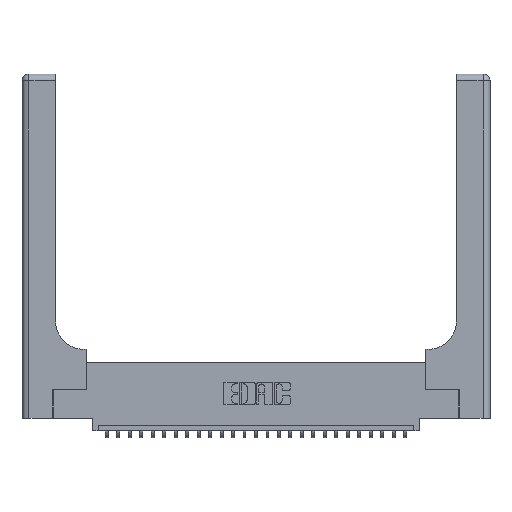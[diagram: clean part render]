
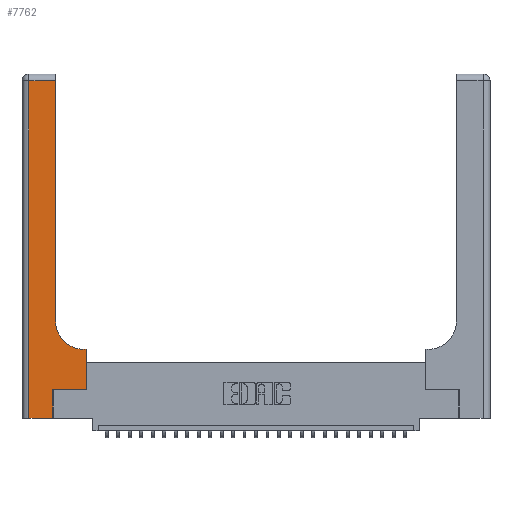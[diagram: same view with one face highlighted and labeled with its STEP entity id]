
A CAD part, top view. The second image highlights one B-rep face of the part: STEP entity #7762.
In plain terms, the highlighted planar face has unit normal (0, 0, 1).
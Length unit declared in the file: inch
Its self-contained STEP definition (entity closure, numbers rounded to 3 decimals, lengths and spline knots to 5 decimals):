
#159 = ORIENTED_EDGE ( 'NONE', *, *, #10812, .T. ) ;
#178 = LINE ( 'NONE', #2615, #13215 ) ;
#665 = ORIENTED_EDGE ( 'NONE', *, *, #11935, .T. ) ;
#1028 = VERTEX_POINT ( 'NONE', #15979 ) ;
#1153 = CARTESIAN_POINT ( 'NONE',  ( 0.2915, 0.85, 0.37 ) ) ;
#2338 = CARTESIAN_POINT ( 'NONE',  ( 0.5585, 0.25, 0.37 ) ) ;
#2615 = CARTESIAN_POINT ( 'NONE',  ( 0.269, 0.25, 0.37 ) ) ;
#2981 = AXIS2_PLACEMENT_3D ( 'NONE', #23404, #27767, #27617 ) ;
#4346 = VECTOR ( 'NONE', #11252, 39.37008 ) ;
#5257 = VERTEX_POINT ( 'NONE', #7479 ) ;
#6535 = EDGE_CURVE ( 'NONE', #14179, #15835, #25869, .T. ) ;
#7274 = ORIENTED_EDGE ( 'NONE', *, *, #15070, .T. ) ;
#7456 = CIRCLE ( 'NONE', #17212, 0.25 ) ;
#7479 = CARTESIAN_POINT ( 'NONE',  ( 0.269, 0.25, 0.37 ) ) ;
#7762 = ADVANCED_FACE ( 'NONE', ( #18041 ), #10646, .F. ) ;
#8376 = VECTOR ( 'NONE', #12177, 39.37008 ) ;
#8519 = CARTESIAN_POINT ( 'NONE',  ( 0.06, 2.94, 0.37 ) ) ;
#8842 = DIRECTION ( 'NONE',  ( 0., -1., 0. ) ) ;
#8872 = LINE ( 'NONE', #14750, #10920 ) ;
#9018 = DIRECTION ( 'NONE',  ( 0., 0., -1. ) ) ;
#9071 = LINE ( 'NONE', #2338, #19741 ) ;
#9731 = LINE ( 'NONE', #22855, #8376 ) ;
#10119 = EDGE_CURVE ( 'NONE', #5257, #11183, #178, .T. ) ;
#10646 = PLANE ( 'NONE',  #2981 ) ;
#10812 = EDGE_CURVE ( 'NONE', #24183, #1028, #15837, .T. ) ;
#10920 = VECTOR ( 'NONE', #12601, 39.37008 ) ;
#10958 = VECTOR ( 'NONE', #27438, 39.37008 ) ;
#11183 = VERTEX_POINT ( 'NONE', #14911 ) ;
#11252 = DIRECTION ( 'NONE',  ( 1., 0., 0. ) ) ;
#11935 = EDGE_CURVE ( 'NONE', #27222, #24183, #7456, .T. ) ;
#12177 = DIRECTION ( 'NONE',  ( -1., 0., 0. ) ) ;
#12399 = DIRECTION ( 'NONE',  ( 0., 1., 0. ) ) ;
#12601 = DIRECTION ( 'NONE',  ( 0., 1., 0. ) ) ;
#12757 = EDGE_CURVE ( 'NONE', #11183, #21862, #9071, .T. ) ;
#13072 = CARTESIAN_POINT ( 'NONE',  ( 0.06, 3., 0.37 ) ) ;
#13200 = EDGE_CURVE ( 'NONE', #1028, #18904, #9731, .T. ) ;
#13215 = VECTOR ( 'NONE', #17261, 39.37008 ) ;
#14179 = VERTEX_POINT ( 'NONE', #22225 ) ;
#14750 = CARTESIAN_POINT ( 'NONE',  ( 0.269, 0., 0.37 ) ) ;
#14891 = ORIENTED_EDGE ( 'NONE', *, *, #12757, .T. ) ;
#14911 = CARTESIAN_POINT ( 'NONE',  ( 0.5585, 0.25, 0.37 ) ) ;
#15070 = EDGE_CURVE ( 'NONE', #21862, #27222, #17313, .T. ) ;
#15089 = DIRECTION ( 'NONE',  ( 0., 1., 0. ) ) ;
#15835 = VERTEX_POINT ( 'NONE', #23240 ) ;
#15837 = LINE ( 'NONE', #21263, #17832 ) ;
#15979 = CARTESIAN_POINT ( 'NONE',  ( 0.2915, 2.94, 0.37 ) ) ;
#16463 = ORIENTED_EDGE ( 'NONE', *, *, #10119, .T. ) ;
#16771 = CARTESIAN_POINT ( 'NONE',  ( 0.5585, 0.6, 0.37 ) ) ;
#17212 = AXIS2_PLACEMENT_3D ( 'NONE', #24038, #9018, #21572 ) ;
#17261 = DIRECTION ( 'NONE',  ( 1., 0., 0. ) ) ;
#17313 = LINE ( 'NONE', #27257, #10958 ) ;
#17832 = VECTOR ( 'NONE', #12399, 39.37008 ) ;
#18011 = CARTESIAN_POINT ( 'NONE',  ( 0.5415, 0.6, 0.37 ) ) ;
#18041 = FACE_OUTER_BOUND ( 'NONE', #23497, .T. ) ;
#18904 = VERTEX_POINT ( 'NONE', #8519 ) ;
#19323 = VECTOR ( 'NONE', #8842, 39.37008 ) ;
#19741 = VECTOR ( 'NONE', #15089, 39.37008 ) ;
#21095 = EDGE_CURVE ( 'NONE', #15835, #5257, #8872, .T. ) ;
#21263 = CARTESIAN_POINT ( 'NONE',  ( 0.2915, 3., 0.37 ) ) ;
#21572 = DIRECTION ( 'NONE',  ( 1., 0., 0. ) ) ;
#21746 = ORIENTED_EDGE ( 'NONE', *, *, #27609, .T. ) ;
#21862 = VERTEX_POINT ( 'NONE', #16771 ) ;
#22225 = CARTESIAN_POINT ( 'NONE',  ( 0.06, 0., 0.37 ) ) ;
#22855 = CARTESIAN_POINT ( 'NONE',  ( 0., 2.94, 0.37 ) ) ;
#23125 = ORIENTED_EDGE ( 'NONE', *, *, #21095, .T. ) ;
#23240 = CARTESIAN_POINT ( 'NONE',  ( 0.269, 0., 0.37 ) ) ;
#23404 = CARTESIAN_POINT ( 'NONE',  ( 0., 3., 0.37 ) ) ;
#23497 = EDGE_LOOP ( 'NONE', ( #159, #24300, #21746, #26240, #23125, #16463, #14891, #7274, #665 ) ) ;
#24038 = CARTESIAN_POINT ( 'NONE',  ( 0.5415, 0.85, 0.37 ) ) ;
#24183 = VERTEX_POINT ( 'NONE', #1153 ) ;
#24196 = CARTESIAN_POINT ( 'NONE',  ( 0., 0., 0.37 ) ) ;
#24300 = ORIENTED_EDGE ( 'NONE', *, *, #13200, .T. ) ;
#24798 = LINE ( 'NONE', #13072, #19323 ) ;
#25869 = LINE ( 'NONE', #24196, #4346 ) ;
#26240 = ORIENTED_EDGE ( 'NONE', *, *, #6535, .T. ) ;
#27222 = VERTEX_POINT ( 'NONE', #18011 ) ;
#27257 = CARTESIAN_POINT ( 'NONE',  ( 0.2915, 0.6, 0.37 ) ) ;
#27438 = DIRECTION ( 'NONE',  ( -1., 0., 0. ) ) ;
#27609 = EDGE_CURVE ( 'NONE', #18904, #14179, #24798, .T. ) ;
#27617 = DIRECTION ( 'NONE',  ( -1., 0., 0. ) ) ;
#27767 = DIRECTION ( 'NONE',  ( 0., 0., -1. ) ) ;
